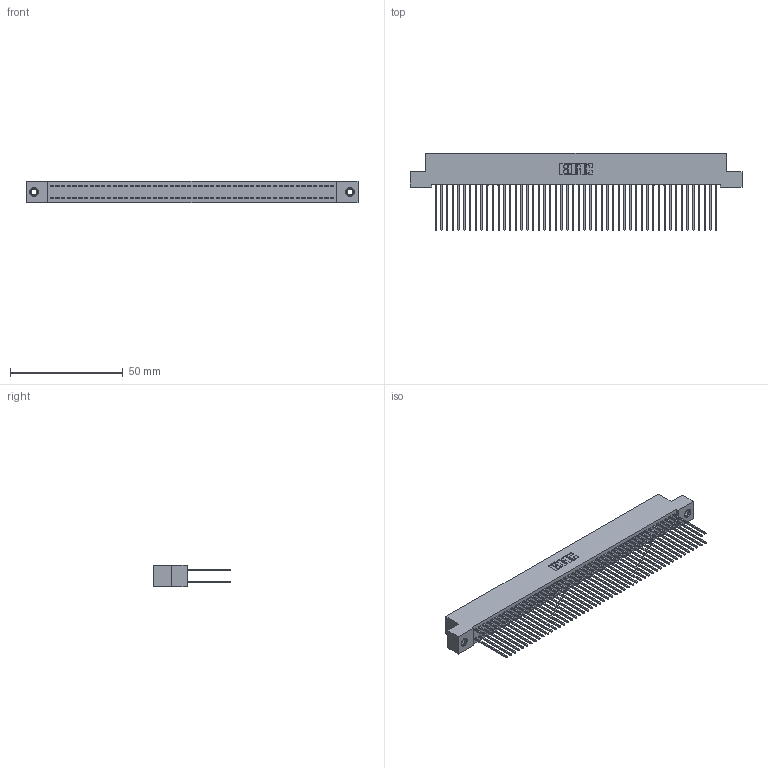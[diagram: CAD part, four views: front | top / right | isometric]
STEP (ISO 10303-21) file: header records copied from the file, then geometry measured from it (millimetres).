
FILE_DESCRIPTION (( 'STEP AP203' ), '1' );
FILE_NAME ('342-100-541-207.STEP', '2018-08-14T04:38:02', ( '' ), ( '' ), 'SwSTEP 2.0', 'SolidWorks 2016', '' );
FILE_SCHEMA (( 'CONFIG_CONTROL_DESIGN' ));
Length unit declared in the file: inch
Products named in the file (4): 342-100-541-207; 342 Part_TI; 345-292-001_345-293-141; 345-250-001_345-250-005-103
Assembly tree (103 placements, depth 2):
  342-100-541-207
    342 Part_TI
    345-292-001_345-293-141  x100
    345-250-001_345-250-005-103  x2
Bounding box: 147.32 x 34.3 x 9.4 mm (x, y, z)
Volume: 13835.6 mm3; surface area: 25338.1 mm2
Topology: 103 solids, 103 shells, 5370 faces, 15935 edges, 10482 vertices
Faces by surface type: plane 3698, cylinder 1656, cone 12, torus 4
Entity records: 32204 total; most frequent: CARTESIAN_POINT 5309, ORIENTED_EDGE 5238, DIRECTION 4553, EDGE_CURVE 2619, LINE 2471, VECTOR 2471, VERTEX_POINT 1740, AXIS2_PLACEMENT_3D 1041
